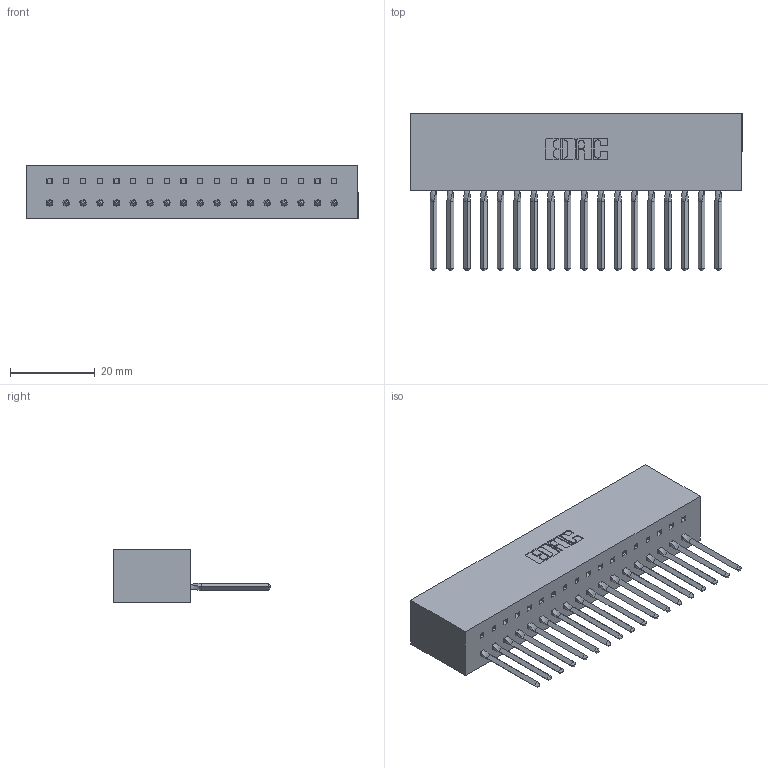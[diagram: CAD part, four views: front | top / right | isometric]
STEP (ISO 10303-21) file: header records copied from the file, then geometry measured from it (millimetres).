
FILE_DESCRIPTION (( 'STEP AP203' ), '1' );
FILE_NAME ('317-018-541-601.STEP', '2020-02-27T15:52:35', ( '' ), ( '' ), 'SwSTEP 2.0', 'SolidWorks 2016', '' );
FILE_SCHEMA (( 'CONFIG_CONTROL_DESIGN' ));
Length unit declared in the file: inch
Products named in the file (3): 317-290-002_541; 317-018-541-601; 317 Part_Lugless
Assembly tree (19 placements, depth 2):
  317-018-541-601
    317 Part_Lugless
    317-290-002_541  x18
Bounding box: 78.54 x 37.34 x 12.7 mm (x, y, z)
Volume: 13703.9 mm3; surface area: 18758 mm2
Topology: 19 solids, 19 shells, 2826 faces, 8051 edges, 5234 vertices
Faces by surface type: plane 2282, cylinder 472, bspline 72
Entity records: 29930 total; most frequent: CARTESIAN_POINT 5951, ORIENTED_EDGE 5222, DIRECTION 4263, EDGE_CURVE 2611, LINE 2255, VECTOR 2255, VERTEX_POINT 1732, AXIS2_PLACEMENT_3D 1004
